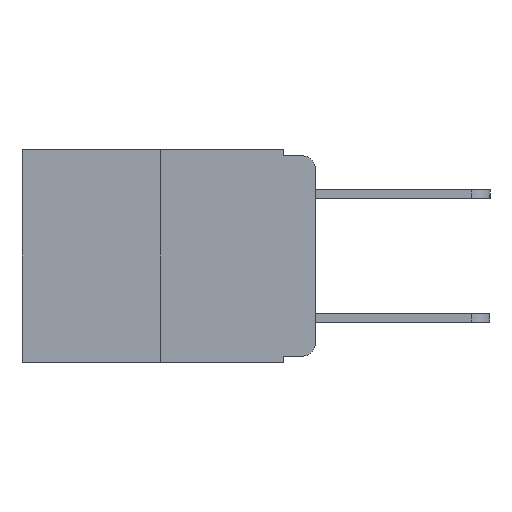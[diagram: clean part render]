
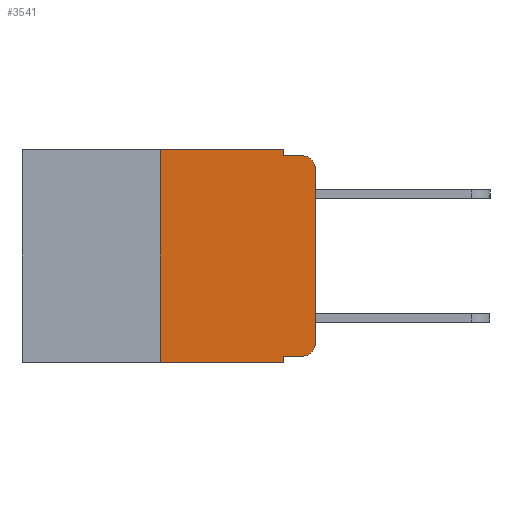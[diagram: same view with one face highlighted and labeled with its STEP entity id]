
A CAD part, left-side view. The second image highlights one B-rep face of the part: STEP entity #3541.
In plain terms, the highlighted planar face has unit normal (-1, 0, 0).
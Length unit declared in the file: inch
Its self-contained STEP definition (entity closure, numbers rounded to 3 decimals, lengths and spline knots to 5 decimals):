
#12 = VECTOR ( 'NONE', #1848, 39.37008 ) ;
#36 = CARTESIAN_POINT ( 'NONE',  ( 0., 0.473, -0.343 ) ) ;
#199 = VECTOR ( 'NONE', #1452, 39.37008 ) ;
#327 = ORIENTED_EDGE ( 'NONE', *, *, #393, .F. ) ;
#393 = EDGE_CURVE ( 'NONE', #6464, #10804, #821, .T. ) ;
#529 = VECTOR ( 'NONE', #560, 39.37008 ) ;
#560 = DIRECTION ( 'NONE',  ( 0., 0., 1. ) ) ;
#633 = CARTESIAN_POINT ( 'NONE',  ( 0., 0.25, 0. ) ) ;
#820 = CARTESIAN_POINT ( 'NONE',  ( 0., 0., -0.03 ) ) ;
#821 = LINE ( 'NONE', #928, #529 ) ;
#928 = CARTESIAN_POINT ( 'NONE',  ( 0., 0.25, 0. ) ) ;
#962 = VECTOR ( 'NONE', #3754, 39.37008 ) ;
#1202 = CARTESIAN_POINT ( 'NONE',  ( 0., 0.051, 0. ) ) ;
#1397 = ORIENTED_EDGE ( 'NONE', *, *, #1779, .F. ) ;
#1452 = DIRECTION ( 'NONE',  ( 0., -1., 0. ) ) ;
#1525 = EDGE_CURVE ( 'NONE', #10804, #7137, #6959, .T. ) ;
#1631 = EDGE_CURVE ( 'NONE', #6464, #3302, #3389, .T. ) ;
#1779 = EDGE_CURVE ( 'NONE', #6714, #3302, #2378, .T. ) ;
#1848 = DIRECTION ( 'NONE',  ( 0., 0., -1. ) ) ;
#2055 = CARTESIAN_POINT ( 'NONE',  ( 0., 0.051, -0.343 ) ) ;
#2247 = ORIENTED_EDGE ( 'NONE', *, *, #1631, .T. ) ;
#2313 = EDGE_CURVE ( 'NONE', #6714, #6103, #6146, .T. ) ;
#2378 = LINE ( 'NONE', #5318, #12 ) ;
#2535 = CARTESIAN_POINT ( 'NONE',  ( 0., 0.051, -0.333 ) ) ;
#2603 = DIRECTION ( 'NONE',  ( 0., -1., 0. ) ) ;
#2609 = EDGE_CURVE ( 'NONE', #6103, #4526, #5445, .T. ) ;
#2812 = CARTESIAN_POINT ( 'NONE',  ( 0., 0.02, -0.01 ) ) ;
#2858 = ORIENTED_EDGE ( 'NONE', *, *, #2313, .T. ) ;
#3302 = VERTEX_POINT ( 'NONE', #2055 ) ;
#3312 = AXIS2_PLACEMENT_3D ( 'NONE', #7164, #8540, #5616 ) ;
#3389 = LINE ( 'NONE', #36, #962 ) ;
#3541 = ADVANCED_FACE ( 'NONE', ( #7910 ), #8550, .F. ) ;
#3663 = ORIENTED_EDGE ( 'NONE', *, *, #9047, .T. ) ;
#3677 = VECTOR ( 'NONE', #2603, 39.37008 ) ;
#3754 = DIRECTION ( 'NONE',  ( 0., -1., 0. ) ) ;
#4055 = DIRECTION ( 'NONE',  ( 0., -1., 0. ) ) ;
#4156 = CARTESIAN_POINT ( 'NONE',  ( 0., 0.473, 0. ) ) ;
#4526 = VERTEX_POINT ( 'NONE', #10004 ) ;
#4566 = VECTOR ( 'NONE', #4055, 39.37008 ) ;
#4750 = EDGE_CURVE ( 'NONE', #7137, #10658, #9724, .T. ) ;
#4980 = CARTESIAN_POINT ( 'NONE',  ( 0., 0.25, -0.343 ) ) ;
#5146 = EDGE_CURVE ( 'NONE', #10658, #7315, #7395, .T. ) ;
#5186 = VERTEX_POINT ( 'NONE', #820 ) ;
#5194 = CARTESIAN_POINT ( 'NONE',  ( 0., 0.051, -0.01 ) ) ;
#5318 = CARTESIAN_POINT ( 'NONE',  ( 0., 0.051, 0. ) ) ;
#5445 = CIRCLE ( 'NONE', #8816, 0.02 ) ;
#5616 = DIRECTION ( 'NONE',  ( 0., 0., -1. ) ) ;
#6103 = VERTEX_POINT ( 'NONE', #10940 ) ;
#6146 = LINE ( 'NONE', #2535, #3677 ) ;
#6168 = ORIENTED_EDGE ( 'NONE', *, *, #10565, .T. ) ;
#6464 = VERTEX_POINT ( 'NONE', #4980 ) ;
#6468 = AXIS2_PLACEMENT_3D ( 'NONE', #6585, #6471, #6584 ) ;
#6471 = DIRECTION ( 'NONE',  ( -1., 0., 0. ) ) ;
#6584 = DIRECTION ( 'NONE',  ( 0., 0., -1. ) ) ;
#6585 = CARTESIAN_POINT ( 'NONE',  ( 0., 0.02, -0.03 ) ) ;
#6671 = CARTESIAN_POINT ( 'NONE',  ( 0., 0., 0. ) ) ;
#6714 = VERTEX_POINT ( 'NONE', #10256 ) ;
#6953 = CARTESIAN_POINT ( 'NONE',  ( 0., 0.051, 0. ) ) ;
#6959 = LINE ( 'NONE', #4156, #4566 ) ;
#6991 = EDGE_LOOP ( 'NONE', ( #6168, #3663, #7296, #7932, #10481, #327, #2247, #1397, #2858, #10014 ) ) ;
#7137 = VERTEX_POINT ( 'NONE', #1202 ) ;
#7164 = CARTESIAN_POINT ( 'NONE',  ( 0., 0.473, 0. ) ) ;
#7296 = ORIENTED_EDGE ( 'NONE', *, *, #5146, .F. ) ;
#7315 = VERTEX_POINT ( 'NONE', #2812 ) ;
#7395 = LINE ( 'NONE', #5194, #199 ) ;
#7401 = VECTOR ( 'NONE', #8190, 39.37008 ) ;
#7583 = VECTOR ( 'NONE', #8240, 39.37008 ) ;
#7827 = LINE ( 'NONE', #6671, #7583 ) ;
#7910 = FACE_OUTER_BOUND ( 'NONE', #6991, .T. ) ;
#7932 = ORIENTED_EDGE ( 'NONE', *, *, #4750, .F. ) ;
#8190 = DIRECTION ( 'NONE',  ( 0., 0., -1. ) ) ;
#8240 = DIRECTION ( 'NONE',  ( 0., 0., 1. ) ) ;
#8540 = DIRECTION ( 'NONE',  ( 1., 0., 0. ) ) ;
#8550 = PLANE ( 'NONE',  #3312 ) ;
#8600 = CIRCLE ( 'NONE', #6468, 0.02 ) ;
#8816 = AXIS2_PLACEMENT_3D ( 'NONE', #9116, #9103, #8995 ) ;
#8995 = DIRECTION ( 'NONE',  ( 0., 0., -1. ) ) ;
#9047 = EDGE_CURVE ( 'NONE', #5186, #7315, #8600, .T. ) ;
#9103 = DIRECTION ( 'NONE',  ( -1., 0., 0. ) ) ;
#9116 = CARTESIAN_POINT ( 'NONE',  ( 0., 0.02, -0.313 ) ) ;
#9177 = CARTESIAN_POINT ( 'NONE',  ( 0., 0.051, -0.01 ) ) ;
#9724 = LINE ( 'NONE', #6953, #7401 ) ;
#10004 = CARTESIAN_POINT ( 'NONE',  ( 0., 0., -0.313 ) ) ;
#10014 = ORIENTED_EDGE ( 'NONE', *, *, #2609, .T. ) ;
#10256 = CARTESIAN_POINT ( 'NONE',  ( 0., 0.051, -0.333 ) ) ;
#10481 = ORIENTED_EDGE ( 'NONE', *, *, #1525, .F. ) ;
#10565 = EDGE_CURVE ( 'NONE', #4526, #5186, #7827, .T. ) ;
#10658 = VERTEX_POINT ( 'NONE', #9177 ) ;
#10804 = VERTEX_POINT ( 'NONE', #633 ) ;
#10940 = CARTESIAN_POINT ( 'NONE',  ( 0., 0.02, -0.333 ) ) ;
